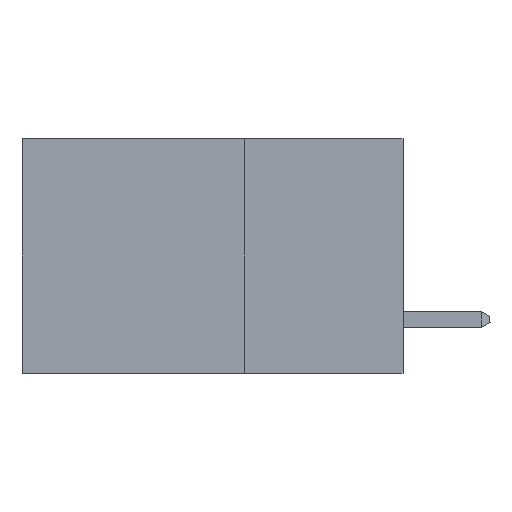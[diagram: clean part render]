
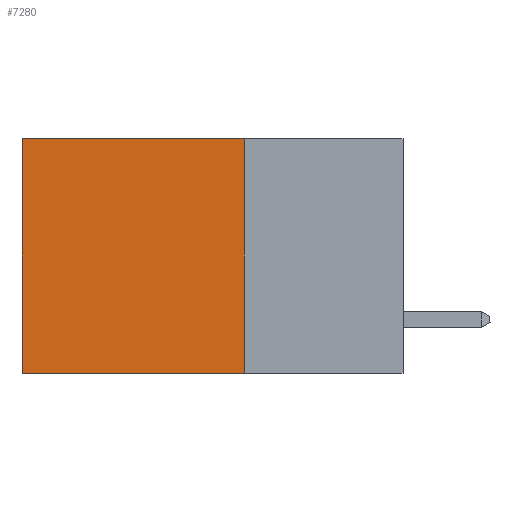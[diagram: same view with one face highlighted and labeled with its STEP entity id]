
A CAD part, left-side view. The second image highlights one B-rep face of the part: STEP entity #7280.
In plain terms, the highlighted planar face has unit normal (-1, 0, 0).
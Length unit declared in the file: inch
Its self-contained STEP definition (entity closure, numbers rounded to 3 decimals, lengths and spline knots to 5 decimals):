
#73 = VERTEX_POINT ( 'NONE', #883 ) ;
#296 = AXIS2_PLACEMENT_3D ( 'NONE', #8795, #5764, #1177 ) ;
#883 = CARTESIAN_POINT ( 'NONE',  ( 0.2875, 0.25, 0. ) ) ;
#992 = ORIENTED_EDGE ( 'NONE', *, *, #2233, .F. ) ;
#1177 = DIRECTION ( 'NONE',  ( 0., 0., -1. ) ) ;
#1285 = DIRECTION ( 'NONE',  ( 0., 1., 0. ) ) ;
#1291 = EDGE_LOOP ( 'NONE', ( #3712, #7244, #992, #3587 ) ) ;
#1507 = LINE ( 'NONE', #6606, #9475 ) ;
#1560 = CARTESIAN_POINT ( 'NONE',  ( 0.2875, 0.6, 0. ) ) ;
#1869 = LINE ( 'NONE', #1560, #3415 ) ;
#1944 = PLANE ( 'NONE',  #296 ) ;
#2233 = EDGE_CURVE ( 'NONE', #73, #2274, #3654, .T. ) ;
#2274 = VERTEX_POINT ( 'NONE', #4665 ) ;
#2385 = EDGE_CURVE ( 'NONE', #5192, #6943, #1869, .T. ) ;
#2461 = VECTOR ( 'NONE', #6775, 39.37008 ) ;
#2898 = CARTESIAN_POINT ( 'NONE',  ( 0.2875, 0.6, -0.37 ) ) ;
#3120 = FACE_OUTER_BOUND ( 'NONE', #1291, .T. ) ;
#3415 = VECTOR ( 'NONE', #7787, 39.37008 ) ;
#3587 = ORIENTED_EDGE ( 'NONE', *, *, #8289, .T. ) ;
#3654 = LINE ( 'NONE', #4499, #2461 ) ;
#3712 = ORIENTED_EDGE ( 'NONE', *, *, #2385, .T. ) ;
#4183 = VECTOR ( 'NONE', #1285, 39.37008 ) ;
#4499 = CARTESIAN_POINT ( 'NONE',  ( 0.2875, 0.25, 0. ) ) ;
#4665 = CARTESIAN_POINT ( 'NONE',  ( 0.2875, 0.25, -0.37 ) ) ;
#5192 = VERTEX_POINT ( 'NONE', #6213 ) ;
#5764 = DIRECTION ( 'NONE',  ( 1., 0., 0. ) ) ;
#5907 = CARTESIAN_POINT ( 'NONE',  ( 0.2875, 0.25, 0. ) ) ;
#6213 = CARTESIAN_POINT ( 'NONE',  ( 0.2875, 0.6, 0. ) ) ;
#6284 = DIRECTION ( 'NONE',  ( 0., 1., 0. ) ) ;
#6606 = CARTESIAN_POINT ( 'NONE',  ( 0.2875, 0.25, -0.37 ) ) ;
#6775 = DIRECTION ( 'NONE',  ( 0., 0., -1. ) ) ;
#6943 = VERTEX_POINT ( 'NONE', #2898 ) ;
#7244 = ORIENTED_EDGE ( 'NONE', *, *, #8972, .F. ) ;
#7280 = ADVANCED_FACE ( 'NONE', ( #3120 ), #1944, .F. ) ;
#7787 = DIRECTION ( 'NONE',  ( 0., 0., -1. ) ) ;
#8289 = EDGE_CURVE ( 'NONE', #73, #5192, #9843, .T. ) ;
#8795 = CARTESIAN_POINT ( 'NONE',  ( 0.2875, 0.25, 0. ) ) ;
#8972 = EDGE_CURVE ( 'NONE', #2274, #6943, #1507, .T. ) ;
#9475 = VECTOR ( 'NONE', #6284, 39.37008 ) ;
#9843 = LINE ( 'NONE', #5907, #4183 ) ;
